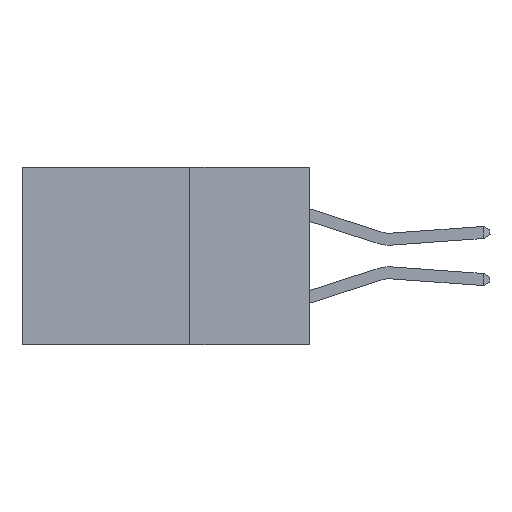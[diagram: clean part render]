
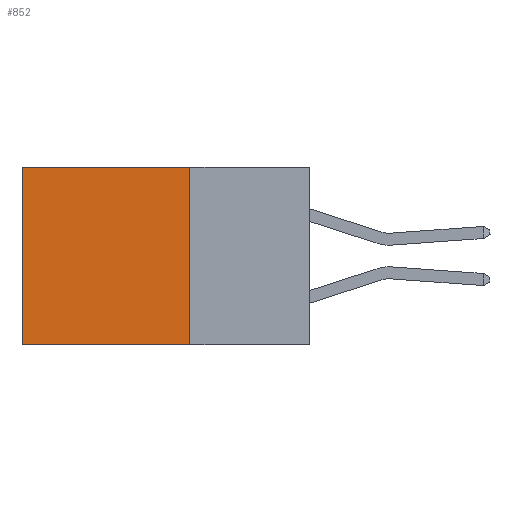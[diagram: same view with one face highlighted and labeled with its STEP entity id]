
A CAD part, left-side view. The second image highlights one B-rep face of the part: STEP entity #852.
In plain terms, the highlighted planar face has unit normal (-1, 0, 0).
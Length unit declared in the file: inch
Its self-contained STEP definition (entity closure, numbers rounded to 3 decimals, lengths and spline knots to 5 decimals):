
#545 = CARTESIAN_POINT ( 'NONE',  ( 0.2615, 0.6, 0. ) ) ;
#550 = EDGE_CURVE ( 'NONE', #3871, #4475, #1207, .T. ) ;
#852 = ADVANCED_FACE ( 'NONE', ( #8096 ), #3962, .F. ) ;
#957 = VECTOR ( 'NONE', #6341, 39.37008 ) ;
#1207 = LINE ( 'NONE', #3387, #957 ) ;
#1618 = ORIENTED_EDGE ( 'NONE', *, *, #6728, .F. ) ;
#1660 = VERTEX_POINT ( 'NONE', #545 ) ;
#1786 = LINE ( 'NONE', #2940, #8811 ) ;
#1798 = CARTESIAN_POINT ( 'NONE',  ( 0.2615, 0.25, 0. ) ) ;
#2250 = DIRECTION ( 'NONE',  ( 0., 1., 0. ) ) ;
#2599 = AXIS2_PLACEMENT_3D ( 'NONE', #7497, #5865, #4303 ) ;
#2616 = CARTESIAN_POINT ( 'NONE',  ( 0.2615, 0.25, -0.37 ) ) ;
#2940 = CARTESIAN_POINT ( 'NONE',  ( 0.2615, 0.25, 0. ) ) ;
#3174 = LINE ( 'NONE', #8549, #3385 ) ;
#3385 = VECTOR ( 'NONE', #4490, 39.37008 ) ;
#3387 = CARTESIAN_POINT ( 'NONE',  ( 0.2615, 0.25, -0.37 ) ) ;
#3573 = DIRECTION ( 'NONE',  ( 0., 1., 0. ) ) ;
#3871 = VERTEX_POINT ( 'NONE', #1798 ) ;
#3884 = ORIENTED_EDGE ( 'NONE', *, *, #5862, .T. ) ;
#3962 = PLANE ( 'NONE',  #2599 ) ;
#4303 = DIRECTION ( 'NONE',  ( 0., 0., -1. ) ) ;
#4475 = VERTEX_POINT ( 'NONE', #2616 ) ;
#4490 = DIRECTION ( 'NONE',  ( 0., 0., -1. ) ) ;
#4809 = CARTESIAN_POINT ( 'NONE',  ( 0.2615, 0.6, -0.37 ) ) ;
#5065 = ORIENTED_EDGE ( 'NONE', *, *, #7167, .T. ) ;
#5557 = VECTOR ( 'NONE', #3573, 39.37008 ) ;
#5862 = EDGE_CURVE ( 'NONE', #3871, #1660, #1786, .T. ) ;
#5865 = DIRECTION ( 'NONE',  ( 1., 0., 0. ) ) ;
#6341 = DIRECTION ( 'NONE',  ( 0., 0., -1. ) ) ;
#6516 = VERTEX_POINT ( 'NONE', #4809 ) ;
#6708 = EDGE_LOOP ( 'NONE', ( #5065, #1618, #7324, #3884 ) ) ;
#6728 = EDGE_CURVE ( 'NONE', #4475, #6516, #9093, .T. ) ;
#7167 = EDGE_CURVE ( 'NONE', #1660, #6516, #3174, .T. ) ;
#7324 = ORIENTED_EDGE ( 'NONE', *, *, #550, .F. ) ;
#7497 = CARTESIAN_POINT ( 'NONE',  ( 0.2615, 0.25, -0.37 ) ) ;
#8096 = FACE_OUTER_BOUND ( 'NONE', #6708, .T. ) ;
#8549 = CARTESIAN_POINT ( 'NONE',  ( 0.2615, 0.6, -0.37 ) ) ;
#8811 = VECTOR ( 'NONE', #2250, 39.37008 ) ;
#8959 = CARTESIAN_POINT ( 'NONE',  ( 0.2615, 0.25, -0.37 ) ) ;
#9093 = LINE ( 'NONE', #8959, #5557 ) ;
